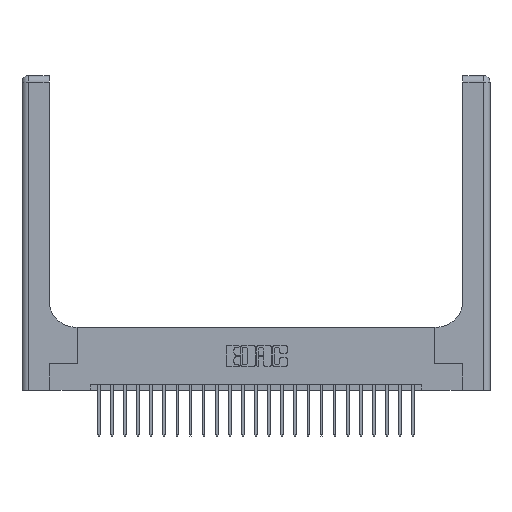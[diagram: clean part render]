
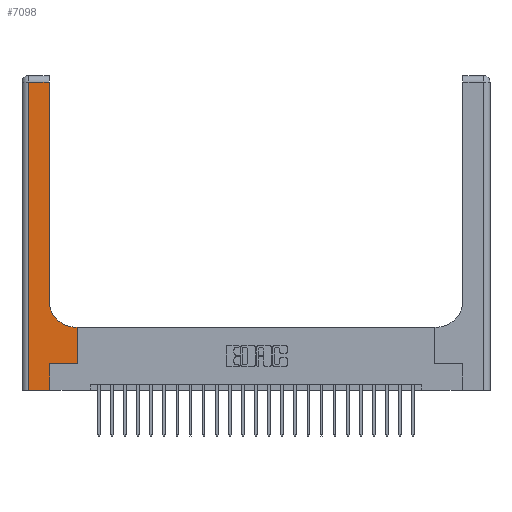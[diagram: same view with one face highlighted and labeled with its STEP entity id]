
A CAD part, top view. The second image highlights one B-rep face of the part: STEP entity #7098.
In plain terms, the highlighted planar face has unit normal (0, 0, 1).
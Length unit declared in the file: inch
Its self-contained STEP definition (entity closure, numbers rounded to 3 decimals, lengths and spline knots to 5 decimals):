
#546 = CARTESIAN_POINT ( 'NONE',  ( 0.06, 3., 0.37 ) ) ;
#861 = CARTESIAN_POINT ( 'NONE',  ( 0.265, 0., 0.37 ) ) ;
#1367 = DIRECTION ( 'NONE',  ( 0., 0., -1. ) ) ;
#1951 = ORIENTED_EDGE ( 'NONE', *, *, #6224, .T. ) ;
#2277 = EDGE_CURVE ( 'NONE', #3400, #7542, #16031, .T. ) ;
#2374 = EDGE_CURVE ( 'NONE', #18775, #20272, #10551, .T. ) ;
#2508 = ORIENTED_EDGE ( 'NONE', *, *, #2374, .T. ) ;
#3143 = CARTESIAN_POINT ( 'NONE',  ( 0.26, 2.94, 0.37 ) ) ;
#3400 = VERTEX_POINT ( 'NONE', #11761 ) ;
#3557 = CARTESIAN_POINT ( 'NONE',  ( 0.265, 0.25, 0.37 ) ) ;
#4442 = PLANE ( 'NONE',  #22052 ) ;
#4593 = FACE_OUTER_BOUND ( 'NONE', #16362, .T. ) ;
#4610 = DIRECTION ( 'NONE',  ( -1., 0., 0. ) ) ;
#4634 = CARTESIAN_POINT ( 'NONE',  ( 0., 2.94, 0.37 ) ) ;
#4998 = CARTESIAN_POINT ( 'NONE',  ( 0.51, 0.85, 0.37 ) ) ;
#5296 = LINE ( 'NONE', #546, #13279 ) ;
#5320 = ORIENTED_EDGE ( 'NONE', *, *, #11091, .T. ) ;
#6224 = EDGE_CURVE ( 'NONE', #13855, #12797, #5296, .T. ) ;
#6564 = VECTOR ( 'NONE', #19547, 39.37008 ) ;
#6597 = CARTESIAN_POINT ( 'NONE',  ( 0.06, 2.94, 0.37 ) ) ;
#6870 = LINE ( 'NONE', #4634, #13699 ) ;
#6879 = DIRECTION ( 'NONE',  ( 1., 0., 0. ) ) ;
#6946 = VECTOR ( 'NONE', #20358, 39.37008 ) ;
#6984 = CARTESIAN_POINT ( 'NONE',  ( 0.528, 0.25, 0.37 ) ) ;
#7004 = LINE ( 'NONE', #861, #7592 ) ;
#7098 = ADVANCED_FACE ( 'NONE', ( #4593 ), #4442, .F. ) ;
#7366 = AXIS2_PLACEMENT_3D ( 'NONE', #4998, #1367, #19451 ) ;
#7535 = EDGE_CURVE ( 'NONE', #10488, #13855, #6870, .T. ) ;
#7542 = VERTEX_POINT ( 'NONE', #23256 ) ;
#7551 = ORIENTED_EDGE ( 'NONE', *, *, #13361, .T. ) ;
#7592 = VECTOR ( 'NONE', #17406, 39.37008 ) ;
#7844 = ORIENTED_EDGE ( 'NONE', *, *, #23243, .T. ) ;
#9170 = VECTOR ( 'NONE', #6879, 39.37008 ) ;
#10488 = VERTEX_POINT ( 'NONE', #3143 ) ;
#10551 = CIRCLE ( 'NONE', #7366, 0.25 ) ;
#11091 = EDGE_CURVE ( 'NONE', #11905, #3400, #7004, .T. ) ;
#11195 = ORIENTED_EDGE ( 'NONE', *, *, #12610, .T. ) ;
#11521 = ORIENTED_EDGE ( 'NONE', *, *, #2277, .T. ) ;
#11542 = DIRECTION ( 'NONE',  ( 0., 0., -1. ) ) ;
#11703 = CARTESIAN_POINT ( 'NONE',  ( 0., 3., 0.37 ) ) ;
#11751 = DIRECTION ( 'NONE',  ( 0., -1., 0. ) ) ;
#11761 = CARTESIAN_POINT ( 'NONE',  ( 0.265, 0.25, 0.37 ) ) ;
#11852 = ORIENTED_EDGE ( 'NONE', *, *, #7535, .T. ) ;
#11905 = VERTEX_POINT ( 'NONE', #21912 ) ;
#11927 = CARTESIAN_POINT ( 'NONE',  ( 0.06, 0., 0.37 ) ) ;
#12084 = LINE ( 'NONE', #22051, #6946 ) ;
#12610 = EDGE_CURVE ( 'NONE', #14006, #18775, #12084, .T. ) ;
#12768 = VECTOR ( 'NONE', #22576, 39.37008 ) ;
#12797 = VERTEX_POINT ( 'NONE', #11927 ) ;
#13279 = VECTOR ( 'NONE', #11751, 39.37008 ) ;
#13361 = EDGE_CURVE ( 'NONE', #20272, #10488, #21991, .T. ) ;
#13699 = VECTOR ( 'NONE', #19698, 39.37008 ) ;
#13855 = VERTEX_POINT ( 'NONE', #6597 ) ;
#13956 = CARTESIAN_POINT ( 'NONE',  ( 0.26, 0.85, 0.37 ) ) ;
#14006 = VERTEX_POINT ( 'NONE', #21455 ) ;
#14042 = CARTESIAN_POINT ( 'NONE',  ( 0.26, 3., 0.37 ) ) ;
#14977 = CARTESIAN_POINT ( 'NONE',  ( 0.51, 0.6, 0.37 ) ) ;
#16031 = LINE ( 'NONE', #3557, #9170 ) ;
#16362 = EDGE_LOOP ( 'NONE', ( #7551, #11852, #1951, #7844, #5320, #11521, #21142, #11195, #2508 ) ) ;
#16997 = CARTESIAN_POINT ( 'NONE',  ( 0., 0., 0.37 ) ) ;
#17406 = DIRECTION ( 'NONE',  ( 0., 1., 0. ) ) ;
#18775 = VERTEX_POINT ( 'NONE', #14977 ) ;
#19451 = DIRECTION ( 'NONE',  ( 1., 0., 0. ) ) ;
#19518 = LINE ( 'NONE', #6984, #23539 ) ;
#19547 = DIRECTION ( 'NONE',  ( 0., 1., 0. ) ) ;
#19698 = DIRECTION ( 'NONE',  ( -1., 0., 0. ) ) ;
#20272 = VERTEX_POINT ( 'NONE', #13956 ) ;
#20358 = DIRECTION ( 'NONE',  ( -1., 0., 0. ) ) ;
#20890 = EDGE_CURVE ( 'NONE', #7542, #14006, #19518, .T. ) ;
#20908 = LINE ( 'NONE', #16997, #12768 ) ;
#21142 = ORIENTED_EDGE ( 'NONE', *, *, #20890, .T. ) ;
#21455 = CARTESIAN_POINT ( 'NONE',  ( 0.528, 0.6, 0.37 ) ) ;
#21783 = DIRECTION ( 'NONE',  ( 0., 1., 0. ) ) ;
#21912 = CARTESIAN_POINT ( 'NONE',  ( 0.265, 0., 0.37 ) ) ;
#21991 = LINE ( 'NONE', #14042, #6564 ) ;
#22051 = CARTESIAN_POINT ( 'NONE',  ( 0.26, 0.6, 0.37 ) ) ;
#22052 = AXIS2_PLACEMENT_3D ( 'NONE', #11703, #11542, #4610 ) ;
#22576 = DIRECTION ( 'NONE',  ( 1., 0., 0. ) ) ;
#23243 = EDGE_CURVE ( 'NONE', #12797, #11905, #20908, .T. ) ;
#23256 = CARTESIAN_POINT ( 'NONE',  ( 0.528, 0.25, 0.37 ) ) ;
#23539 = VECTOR ( 'NONE', #21783, 39.37008 ) ;
